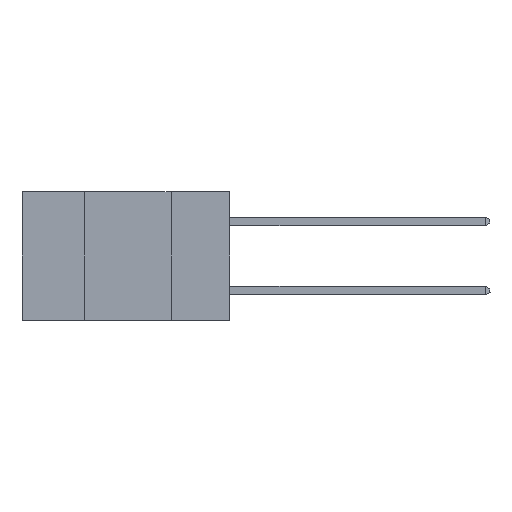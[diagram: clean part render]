
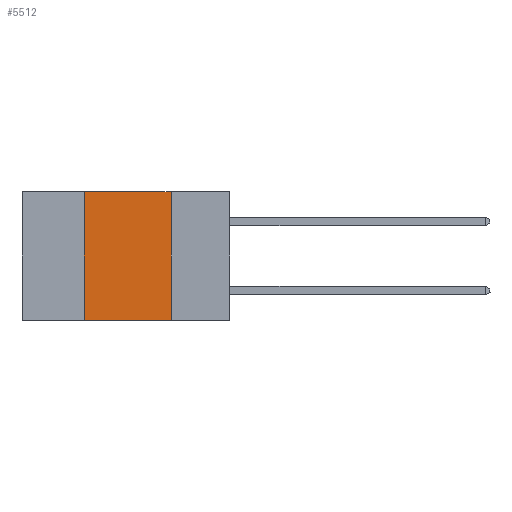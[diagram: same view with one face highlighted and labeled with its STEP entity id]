
A CAD part, left-side view. The second image highlights one B-rep face of the part: STEP entity #5512.
In plain terms, the highlighted planar face has unit normal (-1, 0, 0).
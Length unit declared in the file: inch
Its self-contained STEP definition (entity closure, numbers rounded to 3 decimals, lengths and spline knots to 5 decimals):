
#156 = ORIENTED_EDGE ( 'NONE', *, *, #1395, .F. ) ;
#787 = CARTESIAN_POINT ( 'NONE',  ( 0., 0.42, -0.37 ) ) ;
#1122 = VECTOR ( 'NONE', #13565, 39.37008 ) ;
#1395 = EDGE_CURVE ( 'NONE', #27460, #28788, #14434, .T. ) ;
#3672 = EDGE_CURVE ( 'NONE', #22234, #21355, #29997, .T. ) ;
#5143 = DIRECTION ( 'NONE',  ( 0., 0., 1. ) ) ;
#5173 = CARTESIAN_POINT ( 'NONE',  ( 0., 0.6, 0. ) ) ;
#5512 = ADVANCED_FACE ( 'NONE', ( #23414 ), #11977, .F. ) ;
#5627 = VECTOR ( 'NONE', #31343, 39.37008 ) ;
#6970 = CARTESIAN_POINT ( 'NONE',  ( 0., 0.17, -0.37 ) ) ;
#7058 = LINE ( 'NONE', #5173, #1122 ) ;
#7600 = VECTOR ( 'NONE', #5143, 39.37008 ) ;
#11977 = PLANE ( 'NONE',  #33174 ) ;
#13565 = DIRECTION ( 'NONE',  ( 0., -1., 0. ) ) ;
#14434 = LINE ( 'NONE', #25983, #7600 ) ;
#14532 = DIRECTION ( 'NONE',  ( 0., 0., -1. ) ) ;
#14785 = ORIENTED_EDGE ( 'NONE', *, *, #18291, .F. ) ;
#18291 = EDGE_CURVE ( 'NONE', #28788, #22234, #7058, .T. ) ;
#19035 = CARTESIAN_POINT ( 'NONE',  ( 0., 0.17, 0. ) ) ;
#19956 = CARTESIAN_POINT ( 'NONE',  ( 0., 0.6, 0. ) ) ;
#21035 = EDGE_CURVE ( 'NONE', #27460, #21355, #26905, .T. ) ;
#21036 = CARTESIAN_POINT ( 'NONE',  ( 0., 0.6, -0.37 ) ) ;
#21255 = EDGE_LOOP ( 'NONE', ( #31751, #14785, #156, #29372 ) ) ;
#21355 = VERTEX_POINT ( 'NONE', #6970 ) ;
#21543 = VECTOR ( 'NONE', #14532, 39.37008 ) ;
#22234 = VERTEX_POINT ( 'NONE', #19035 ) ;
#22393 = DIRECTION ( 'NONE',  ( 0., 0., -1. ) ) ;
#23414 = FACE_OUTER_BOUND ( 'NONE', #21255, .T. ) ;
#25983 = CARTESIAN_POINT ( 'NONE',  ( 0., 0.42, 0. ) ) ;
#26905 = LINE ( 'NONE', #21036, #5627 ) ;
#27460 = VERTEX_POINT ( 'NONE', #787 ) ;
#28788 = VERTEX_POINT ( 'NONE', #30190 ) ;
#29372 = ORIENTED_EDGE ( 'NONE', *, *, #21035, .T. ) ;
#29792 = CARTESIAN_POINT ( 'NONE',  ( 0., 0.17, 0. ) ) ;
#29913 = DIRECTION ( 'NONE',  ( 1., 0., 0. ) ) ;
#29997 = LINE ( 'NONE', #29792, #21543 ) ;
#30190 = CARTESIAN_POINT ( 'NONE',  ( 0., 0.42, 0. ) ) ;
#31343 = DIRECTION ( 'NONE',  ( 0., -1., 0. ) ) ;
#31751 = ORIENTED_EDGE ( 'NONE', *, *, #3672, .F. ) ;
#33174 = AXIS2_PLACEMENT_3D ( 'NONE', #19956, #29913, #22393 ) ;
